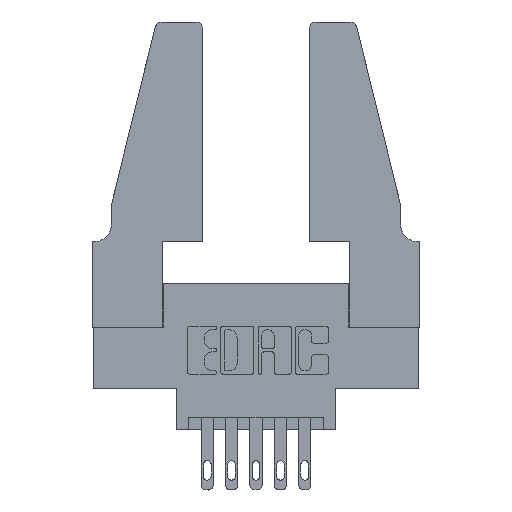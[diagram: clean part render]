
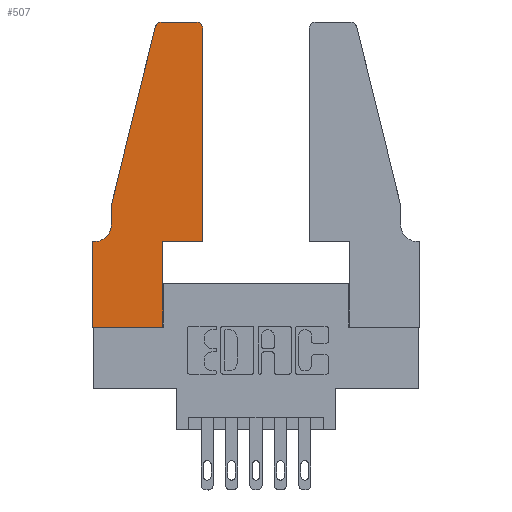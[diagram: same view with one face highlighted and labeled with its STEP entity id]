
A CAD part, top view. The second image highlights one B-rep face of the part: STEP entity #507.
In plain terms, the highlighted planar face has unit normal (0, 0, 1).
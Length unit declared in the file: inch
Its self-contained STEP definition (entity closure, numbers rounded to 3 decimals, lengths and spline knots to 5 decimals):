
#38 = VECTOR ( 'NONE', #2327, 39.37008 ) ;
#126 = DIRECTION ( 'NONE',  ( 0., 0., -1. ) ) ;
#138 = VECTOR ( 'NONE', #3503, 39.37008 ) ;
#182 = VECTOR ( 'NONE', #4044, 39.37008 ) ;
#249 = CIRCLE ( 'NONE', #4932, 0.07 ) ;
#344 = CARTESIAN_POINT ( 'NONE',  ( 0.4205, 1.25, 0.37 ) ) ;
#448 = LINE ( 'NONE', #9186, #182 ) ;
#507 = ADVANCED_FACE ( 'NONE', ( #10245 ), #1649, .T. ) ;
#539 = LINE ( 'NONE', #7311, #9283 ) ;
#578 = EDGE_CURVE ( 'NONE', #2316, #9026, #7002, .T. ) ;
#652 = ORIENTED_EDGE ( 'NONE', *, *, #4698, .T. ) ;
#672 = AXIS2_PLACEMENT_3D ( 'NONE', #10348, #5203, #9408 ) ;
#720 = VERTEX_POINT ( 'NONE', #3317 ) ;
#857 = VERTEX_POINT ( 'NONE', #1066 ) ;
#1066 = CARTESIAN_POINT ( 'NONE',  ( 0.2865, 0.35, 0.37 ) ) ;
#1080 = CARTESIAN_POINT ( 'NONE',  ( 0.0055, 0.42, 0.37 ) ) ;
#1128 = LINE ( 'NONE', #5648, #38 ) ;
#1166 = VERTEX_POINT ( 'NONE', #9274 ) ;
#1269 = VERTEX_POINT ( 'NONE', #7128 ) ;
#1350 = VERTEX_POINT ( 'NONE', #8975 ) ;
#1437 = CARTESIAN_POINT ( 'NONE',  ( 0.0755, 0.42, 0.37 ) ) ;
#1468 = CARTESIAN_POINT ( 'NONE',  ( 0.4205, 1.22, 0.37 ) ) ;
#1649 = PLANE ( 'NONE',  #672 ) ;
#1677 = EDGE_CURVE ( 'NONE', #9026, #857, #7660, .T. ) ;
#1724 = EDGE_CURVE ( 'NONE', #1350, #6294, #539, .T. ) ;
#2316 = VERTEX_POINT ( 'NONE', #7678 ) ;
#2327 = DIRECTION ( 'NONE',  ( -0.239, -0.971, 0. ) ) ;
#2516 = ORIENTED_EDGE ( 'NONE', *, *, #4136, .T. ) ;
#2523 = EDGE_CURVE ( 'NONE', #5397, #1166, #249, .T. ) ;
#2706 = ORIENTED_EDGE ( 'NONE', *, *, #2523, .T. ) ;
#2848 = DIRECTION ( 'NONE',  ( 0., 0., 1. ) ) ;
#3238 = CARTESIAN_POINT ( 'NONE',  ( 0.0755, 0.5, 0.37 ) ) ;
#3317 = CARTESIAN_POINT ( 'NONE',  ( 0.25487, 1.22718, 0.37 ) ) ;
#3503 = DIRECTION ( 'NONE',  ( 0., 1., 0. ) ) ;
#3553 = EDGE_LOOP ( 'NONE', ( #2516, #5467, #3669, #9925, #2706, #10443, #8092, #6188, #4251, #652, #4842, #10953 ) ) ;
#3669 = ORIENTED_EDGE ( 'NONE', *, *, #6034, .T. ) ;
#3801 = CARTESIAN_POINT ( 'NONE',  ( 0.284, 1.22, 0.37 ) ) ;
#3854 = DIRECTION ( 'NONE',  ( 0., 1., 0. ) ) ;
#3864 = VERTEX_POINT ( 'NONE', #4238 ) ;
#4044 = DIRECTION ( 'NONE',  ( -1., 0., 0. ) ) ;
#4134 = CARTESIAN_POINT ( 'NONE',  ( 0., 0.35, 0.37 ) ) ;
#4136 = EDGE_CURVE ( 'NONE', #10892, #3864, #8431, .T. ) ;
#4145 = EDGE_CURVE ( 'NONE', #1269, #5397, #5877, .T. ) ;
#4238 = CARTESIAN_POINT ( 'NONE',  ( 0.284, 1.25, 0.37 ) ) ;
#4251 = ORIENTED_EDGE ( 'NONE', *, *, #1677, .T. ) ;
#4292 = EDGE_CURVE ( 'NONE', #7761, #2316, #10447, .T. ) ;
#4337 = VECTOR ( 'NONE', #10426, 39.37008 ) ;
#4415 = CARTESIAN_POINT ( 'NONE',  ( 0., 0., 0.37 ) ) ;
#4698 = EDGE_CURVE ( 'NONE', #857, #1350, #7066, .T. ) ;
#4734 = CARTESIAN_POINT ( 'NONE',  ( 0.4505, 0.35, 0.37 ) ) ;
#4842 = ORIENTED_EDGE ( 'NONE', *, *, #1724, .T. ) ;
#4920 = DIRECTION ( 'NONE',  ( 0., 0., 1. ) ) ;
#4932 = AXIS2_PLACEMENT_3D ( 'NONE', #1080, #126, #6248 ) ;
#4946 = VECTOR ( 'NONE', #9393, 39.37008 ) ;
#5128 = CARTESIAN_POINT ( 'NONE',  ( 0.2865, 0.35, 0.37 ) ) ;
#5203 = DIRECTION ( 'NONE',  ( 0., 0., 1. ) ) ;
#5397 = VERTEX_POINT ( 'NONE', #1437 ) ;
#5467 = ORIENTED_EDGE ( 'NONE', *, *, #6246, .T. ) ;
#5648 = CARTESIAN_POINT ( 'NONE',  ( 0.0755, 0.5, 0.37 ) ) ;
#5711 = VECTOR ( 'NONE', #6405, 39.37008 ) ;
#5877 = LINE ( 'NONE', #3238, #8956 ) ;
#6034 = EDGE_CURVE ( 'NONE', #720, #1269, #1128, .T. ) ;
#6056 = EDGE_CURVE ( 'NONE', #1166, #7761, #448, .T. ) ;
#6188 = ORIENTED_EDGE ( 'NONE', *, *, #578, .T. ) ;
#6246 = EDGE_CURVE ( 'NONE', #3864, #720, #8507, .T. ) ;
#6248 = DIRECTION ( 'NONE',  ( -1., 0., 0. ) ) ;
#6294 = VERTEX_POINT ( 'NONE', #7206 ) ;
#6405 = DIRECTION ( 'NONE',  ( 1., 0., 0. ) ) ;
#6737 = DIRECTION ( 'NONE',  ( 0., -1., 0. ) ) ;
#6779 = CARTESIAN_POINT ( 'NONE',  ( 0.2605, 1.25, 0.37 ) ) ;
#6787 = DIRECTION ( 'NONE',  ( 0., -1., 0. ) ) ;
#7002 = LINE ( 'NONE', #4415, #4337 ) ;
#7066 = LINE ( 'NONE', #4734, #5711 ) ;
#7128 = CARTESIAN_POINT ( 'NONE',  ( 0.0755, 0.5, 0.37 ) ) ;
#7206 = CARTESIAN_POINT ( 'NONE',  ( 0.4505, 1.22, 0.37 ) ) ;
#7311 = CARTESIAN_POINT ( 'NONE',  ( 0.4505, 0.35, 0.37 ) ) ;
#7449 = AXIS2_PLACEMENT_3D ( 'NONE', #1468, #4920, #9121 ) ;
#7660 = LINE ( 'NONE', #5128, #138 ) ;
#7678 = CARTESIAN_POINT ( 'NONE',  ( 0., 0., 0.37 ) ) ;
#7750 = VECTOR ( 'NONE', #6787, 39.37008 ) ;
#7761 = VERTEX_POINT ( 'NONE', #4134 ) ;
#8092 = ORIENTED_EDGE ( 'NONE', *, *, #4292, .T. ) ;
#8431 = LINE ( 'NONE', #6779, #4946 ) ;
#8507 = CIRCLE ( 'NONE', #10636, 0.03 ) ;
#8797 = CIRCLE ( 'NONE', #7449, 0.03 ) ;
#8956 = VECTOR ( 'NONE', #6737, 39.37008 ) ;
#8975 = CARTESIAN_POINT ( 'NONE',  ( 0.4505, 0.35, 0.37 ) ) ;
#9026 = VERTEX_POINT ( 'NONE', #10464 ) ;
#9094 = DIRECTION ( 'NONE',  ( 1., 0., 0. ) ) ;
#9121 = DIRECTION ( 'NONE',  ( 1., 0., 0. ) ) ;
#9186 = CARTESIAN_POINT ( 'NONE',  ( 0.0755, 0.35, 0.37 ) ) ;
#9274 = CARTESIAN_POINT ( 'NONE',  ( 0.0055, 0.35, 0.37 ) ) ;
#9283 = VECTOR ( 'NONE', #3854, 39.37008 ) ;
#9364 = CARTESIAN_POINT ( 'NONE',  ( 0., 0., 0.37 ) ) ;
#9393 = DIRECTION ( 'NONE',  ( -1., 0., 0. ) ) ;
#9408 = DIRECTION ( 'NONE',  ( 1., 0., 0. ) ) ;
#9853 = EDGE_CURVE ( 'NONE', #6294, #10892, #8797, .T. ) ;
#9925 = ORIENTED_EDGE ( 'NONE', *, *, #4145, .T. ) ;
#10245 = FACE_OUTER_BOUND ( 'NONE', #3553, .T. ) ;
#10348 = CARTESIAN_POINT ( 'NONE',  ( 0., 0.35, 0.37 ) ) ;
#10426 = DIRECTION ( 'NONE',  ( 1., 0., 0. ) ) ;
#10443 = ORIENTED_EDGE ( 'NONE', *, *, #6056, .T. ) ;
#10447 = LINE ( 'NONE', #9364, #7750 ) ;
#10464 = CARTESIAN_POINT ( 'NONE',  ( 0.2865, 0., 0.37 ) ) ;
#10636 = AXIS2_PLACEMENT_3D ( 'NONE', #3801, #2848, #9094 ) ;
#10892 = VERTEX_POINT ( 'NONE', #344 ) ;
#10953 = ORIENTED_EDGE ( 'NONE', *, *, #9853, .T. ) ;
